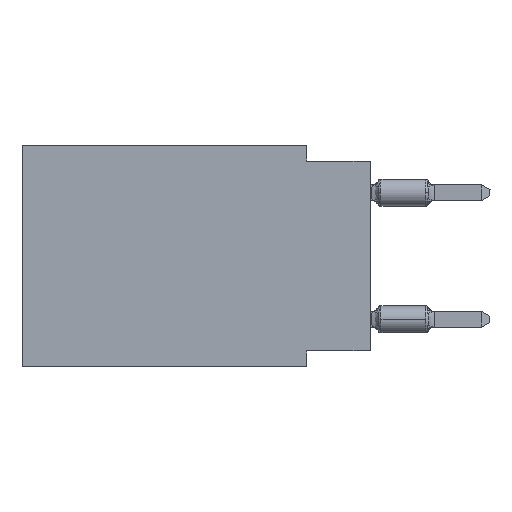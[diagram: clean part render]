
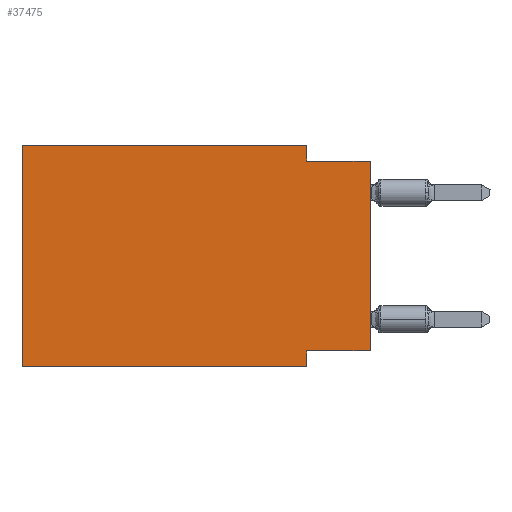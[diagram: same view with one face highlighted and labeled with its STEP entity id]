
A CAD part, left-side view. The second image highlights one B-rep face of the part: STEP entity #37475.
In plain terms, the highlighted planar face has unit normal (-1, 0, 0).
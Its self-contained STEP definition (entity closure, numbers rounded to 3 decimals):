
#843 = VECTOR ( 'NONE', #54534, 1000. ) ;
#1874 = CARTESIAN_POINT ( 'NONE',  ( 0., 2.54, -0.635 ) ) ;
#2970 = LINE ( 'NONE', #64920, #10505 ) ;
#3550 = VERTEX_POINT ( 'NONE', #17349 ) ;
#4703 = CARTESIAN_POINT ( 'NONE',  ( 0., 13.97, -8.89 ) ) ;
#8146 = VERTEX_POINT ( 'NONE', #28900 ) ;
#8802 = DIRECTION ( 'NONE',  ( 0., 0., -1. ) ) ;
#8890 = LINE ( 'NONE', #66059, #52577 ) ;
#9214 = EDGE_CURVE ( 'NONE', #8146, #66133, #9803, .T. ) ;
#9803 = LINE ( 'NONE', #4703, #18866 ) ;
#10169 = ORIENTED_EDGE ( 'NONE', *, *, #57157, .F. ) ;
#10279 = ORIENTED_EDGE ( 'NONE', *, *, #50766, .T. ) ;
#10505 = VECTOR ( 'NONE', #23092, 1000. ) ;
#11779 = ORIENTED_EDGE ( 'NONE', *, *, #18136, .F. ) ;
#13082 = DIRECTION ( 'NONE',  ( 1., 0., 0. ) ) ;
#14393 = ORIENTED_EDGE ( 'NONE', *, *, #9214, .T. ) ;
#14709 = VERTEX_POINT ( 'NONE', #1874 ) ;
#15830 = ORIENTED_EDGE ( 'NONE', *, *, #60473, .F. ) ;
#17349 = CARTESIAN_POINT ( 'NONE',  ( 0., 13.97, 0. ) ) ;
#18136 = EDGE_CURVE ( 'NONE', #43241, #57132, #19084, .T. ) ;
#18866 = VECTOR ( 'NONE', #19687, 1000. ) ;
#19084 = LINE ( 'NONE', #39852, #64374 ) ;
#19514 = FACE_OUTER_BOUND ( 'NONE', #43027, .T. ) ;
#19687 = DIRECTION ( 'NONE',  ( 0., -1., 0. ) ) ;
#23092 = DIRECTION ( 'NONE',  ( 0., -1., 0. ) ) ;
#24098 = VERTEX_POINT ( 'NONE', #64654 ) ;
#24615 = DIRECTION ( 'NONE',  ( 0., 0., -1. ) ) ;
#27285 = LINE ( 'NONE', #44275, #843 ) ;
#28900 = CARTESIAN_POINT ( 'NONE',  ( 0., 13.97, -8.89 ) ) ;
#29044 = PLANE ( 'NONE',  #46013 ) ;
#33410 = DIRECTION ( 'NONE',  ( 0., 0., 1. ) ) ;
#35966 = DIRECTION ( 'NONE',  ( 0., 0., -1. ) ) ;
#36277 = LINE ( 'NONE', #52944, #57501 ) ;
#37475 = ADVANCED_FACE ( 'NONE', ( #19514 ), #29044, .F. ) ;
#37825 = EDGE_CURVE ( 'NONE', #8146, #3550, #8890, .T. ) ;
#38739 = VECTOR ( 'NONE', #35966, 1000. ) ;
#39448 = LINE ( 'NONE', #59887, #57678 ) ;
#39852 = CARTESIAN_POINT ( 'NONE',  ( 0., 0., -8.255 ) ) ;
#43027 = EDGE_LOOP ( 'NONE', ( #10279, #10169, #45203, #56112, #51995, #14393, #15830, #11779 ) ) ;
#43241 = VERTEX_POINT ( 'NONE', #61371 ) ;
#44275 = CARTESIAN_POINT ( 'NONE',  ( 0., 0., -0.635 ) ) ;
#45203 = ORIENTED_EDGE ( 'NONE', *, *, #48074, .F. ) ;
#46013 = AXIS2_PLACEMENT_3D ( 'NONE', #60365, #13082, #24615 ) ;
#46496 = LINE ( 'NONE', #51955, #38739 ) ;
#46925 = CARTESIAN_POINT ( 'NONE',  ( 0., 2.54, -8.89 ) ) ;
#48074 = EDGE_CURVE ( 'NONE', #24098, #14709, #46496, .T. ) ;
#50766 = EDGE_CURVE ( 'NONE', #43241, #65676, #36277, .T. ) ;
#51955 = CARTESIAN_POINT ( 'NONE',  ( 0., 2.54, 0. ) ) ;
#51995 = ORIENTED_EDGE ( 'NONE', *, *, #37825, .F. ) ;
#52103 = CARTESIAN_POINT ( 'NONE',  ( 0., 0., -0.635 ) ) ;
#52577 = VECTOR ( 'NONE', #33410, 1000. ) ;
#52944 = CARTESIAN_POINT ( 'NONE',  ( 0., 0., 0. ) ) ;
#54534 = DIRECTION ( 'NONE',  ( 0., -1., 0. ) ) ;
#54753 = EDGE_CURVE ( 'NONE', #3550, #24098, #2970, .T. ) ;
#56112 = ORIENTED_EDGE ( 'NONE', *, *, #54753, .F. ) ;
#57041 = DIRECTION ( 'NONE',  ( 0., 0., 1. ) ) ;
#57132 = VERTEX_POINT ( 'NONE', #63040 ) ;
#57157 = EDGE_CURVE ( 'NONE', #14709, #65676, #27285, .T. ) ;
#57501 = VECTOR ( 'NONE', #57041, 1000. ) ;
#57678 = VECTOR ( 'NONE', #8802, 1000. ) ;
#59887 = CARTESIAN_POINT ( 'NONE',  ( 0., 2.54, -8.89 ) ) ;
#60365 = CARTESIAN_POINT ( 'NONE',  ( 0., 13.97, 0. ) ) ;
#60473 = EDGE_CURVE ( 'NONE', #57132, #66133, #39448, .T. ) ;
#61371 = CARTESIAN_POINT ( 'NONE',  ( 0., 0., -8.255 ) ) ;
#62444 = DIRECTION ( 'NONE',  ( 0., 1., 0. ) ) ;
#63040 = CARTESIAN_POINT ( 'NONE',  ( 0., 2.54, -8.255 ) ) ;
#64374 = VECTOR ( 'NONE', #62444, 1000. ) ;
#64654 = CARTESIAN_POINT ( 'NONE',  ( 0., 2.54, 0. ) ) ;
#64920 = CARTESIAN_POINT ( 'NONE',  ( 0., 13.97, 0. ) ) ;
#65676 = VERTEX_POINT ( 'NONE', #52103 ) ;
#66059 = CARTESIAN_POINT ( 'NONE',  ( 0., 13.97, 0. ) ) ;
#66133 = VERTEX_POINT ( 'NONE', #46925 ) ;
